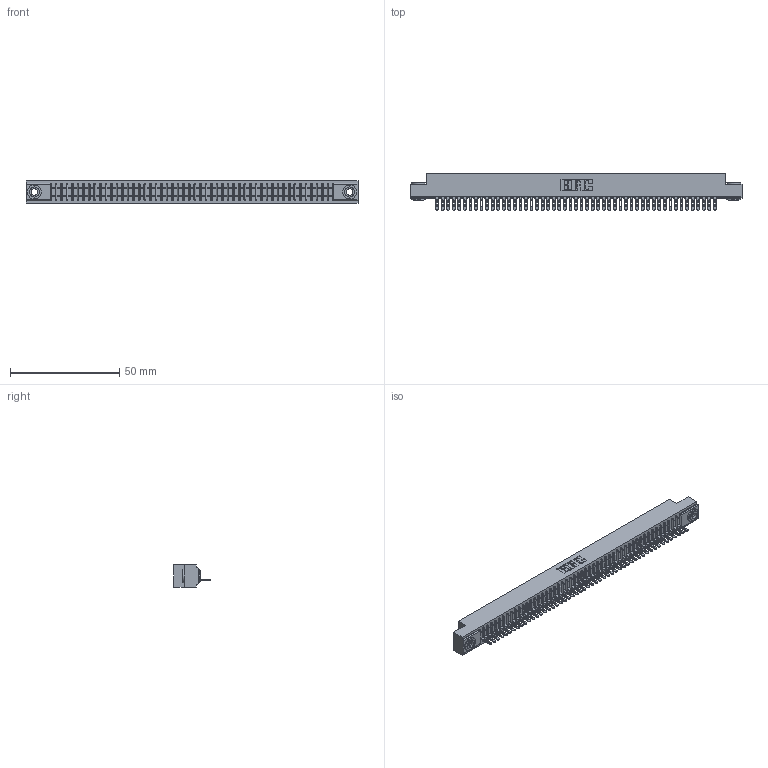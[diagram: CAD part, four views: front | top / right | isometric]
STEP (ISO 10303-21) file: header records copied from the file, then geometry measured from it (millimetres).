
FILE_DESCRIPTION (( 'STEP AP203' ), '1' );
FILE_NAME ('341-051-500-103.STEP', '2018-08-07T12:47:02', ( '' ), ( '' ), 'SwSTEP 2.0', 'SolidWorks 2016', '' );
FILE_SCHEMA (( 'CONFIG_CONTROL_DESIGN' ));
Length unit declared in the file: inch
Products named in the file (4): 341 Part_.156 (3.96) Dia Mounting Holes; 341-292-001_341-292-100; 345-250-002_345-250-002-102; 341-051-500-103
Assembly tree (54 placements, depth 2):
  341-051-500-103
    341 Part_.156 (3.96) Dia Mounting Holes
    341-292-001_341-292-100  x51
    345-250-002_345-250-002-102  x2
Bounding box: 151.76 x 16.69 x 10.16 mm (x, y, z)
Volume: 10917.2 mm3; surface area: 17793.5 mm2
Topology: 54 solids, 54 shells, 4350 faces, 12515 edges, 8030 vertices
Faces by surface type: plane 2591, cylinder 1547, sphere 104, torus 100, cone 8
Entity records: 59963 total; most frequent: CARTESIAN_POINT 10167, ORIENTED_EDGE 10146, DIRECTION 9827, EDGE_CURVE 5073, LINE 4095, VECTOR 4095, VERTEX_POINT 3206, AXIS2_PLACEMENT_3D 2866
